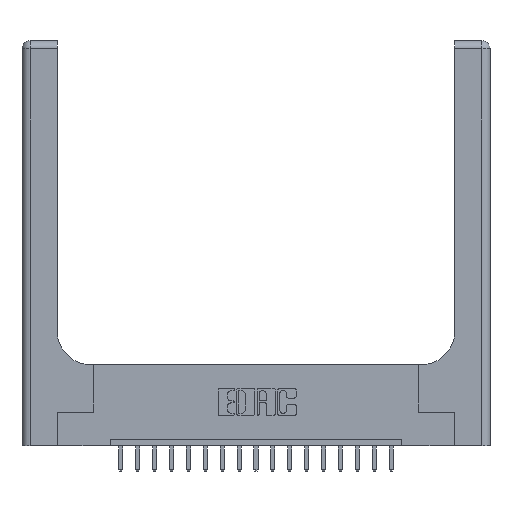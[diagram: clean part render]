
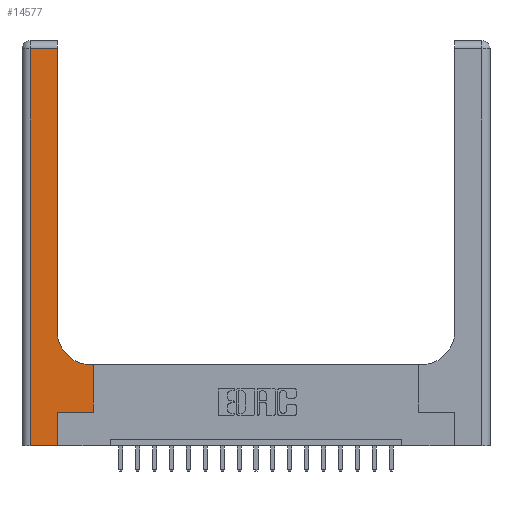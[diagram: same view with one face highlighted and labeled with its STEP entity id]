
A CAD part, top view. The second image highlights one B-rep face of the part: STEP entity #14577.
In plain terms, the highlighted planar face has unit normal (0, 0, 1).
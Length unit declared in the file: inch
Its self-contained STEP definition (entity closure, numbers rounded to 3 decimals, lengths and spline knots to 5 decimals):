
#534 = AXIS2_PLACEMENT_3D ( 'NONE', #12684, #18623, #2195 ) ;
#655 = EDGE_CURVE ( 'NONE', #13978, #4303, #18606, .T. ) ;
#719 = VECTOR ( 'NONE', #15437, 39.37008 ) ;
#831 = CARTESIAN_POINT ( 'NONE',  ( 0.26, 0.85, 0.37 ) ) ;
#1106 = EDGE_CURVE ( 'NONE', #8724, #7962, #4854, .T. ) ;
#1182 = CARTESIAN_POINT ( 'NONE',  ( 0.26, 3., 0.37 ) ) ;
#1614 = VERTEX_POINT ( 'NONE', #3201 ) ;
#1821 = VECTOR ( 'NONE', #2285, 39.37008 ) ;
#1910 = FACE_OUTER_BOUND ( 'NONE', #4806, .T. ) ;
#2195 = DIRECTION ( 'NONE',  ( -1., 0., 0. ) ) ;
#2285 = DIRECTION ( 'NONE',  ( 0., 1., 0. ) ) ;
#2563 = VECTOR ( 'NONE', #13845, 39.37008 ) ;
#2666 = ORIENTED_EDGE ( 'NONE', *, *, #9182, .T. ) ;
#3201 = CARTESIAN_POINT ( 'NONE',  ( 0.26, 2.94, 0.37 ) ) ;
#3688 = CARTESIAN_POINT ( 'NONE',  ( 0.528, 0.25, 0.37 ) ) ;
#3798 = CARTESIAN_POINT ( 'NONE',  ( 0.528, 0.6, 0.37 ) ) ;
#4148 = DIRECTION ( 'NONE',  ( 1., 0., 0. ) ) ;
#4180 = DIRECTION ( 'NONE',  ( 0., 1., 0. ) ) ;
#4295 = AXIS2_PLACEMENT_3D ( 'NONE', #17277, #9638, #14234 ) ;
#4303 = VERTEX_POINT ( 'NONE', #831 ) ;
#4405 = LINE ( 'NONE', #1182, #14149 ) ;
#4723 = CARTESIAN_POINT ( 'NONE',  ( 0.06, 0., 0.37 ) ) ;
#4806 = EDGE_LOOP ( 'NONE', ( #12585, #7739, #9282, #6896, #7894, #6172, #11822, #2666, #18138 ) ) ;
#4854 = LINE ( 'NONE', #11528, #13436 ) ;
#4890 = CARTESIAN_POINT ( 'NONE',  ( 0.06, 3., 0.37 ) ) ;
#4999 = DIRECTION ( 'NONE',  ( 0., 1., 0. ) ) ;
#5219 = EDGE_CURVE ( 'NONE', #8511, #12671, #18846, .T. ) ;
#5603 = EDGE_CURVE ( 'NONE', #11260, #8511, #8600, .T. ) ;
#5658 = CARTESIAN_POINT ( 'NONE',  ( 0.26, 0.6, 0.37 ) ) ;
#6172 = ORIENTED_EDGE ( 'NONE', *, *, #1106, .T. ) ;
#6261 = LINE ( 'NONE', #17069, #1821 ) ;
#6333 = LINE ( 'NONE', #5658, #7228 ) ;
#6896 = ORIENTED_EDGE ( 'NONE', *, *, #5219, .T. ) ;
#6936 = VECTOR ( 'NONE', #14431, 39.37008 ) ;
#7017 = EDGE_CURVE ( 'NONE', #1614, #11260, #9287, .T. ) ;
#7228 = VECTOR ( 'NONE', #19148, 39.37008 ) ;
#7581 = CARTESIAN_POINT ( 'NONE',  ( 0.06, 2.94, 0.37 ) ) ;
#7739 = ORIENTED_EDGE ( 'NONE', *, *, #7017, .T. ) ;
#7894 = ORIENTED_EDGE ( 'NONE', *, *, #15708, .T. ) ;
#7962 = VERTEX_POINT ( 'NONE', #8873 ) ;
#8511 = VERTEX_POINT ( 'NONE', #4723 ) ;
#8600 = LINE ( 'NONE', #4890, #719 ) ;
#8724 = VERTEX_POINT ( 'NONE', #10807 ) ;
#8873 = CARTESIAN_POINT ( 'NONE',  ( 0.528, 0.25, 0.37 ) ) ;
#9137 = VECTOR ( 'NONE', #4999, 39.37008 ) ;
#9182 = EDGE_CURVE ( 'NONE', #11074, #13978, #6333, .T. ) ;
#9282 = ORIENTED_EDGE ( 'NONE', *, *, #5603, .T. ) ;
#9287 = LINE ( 'NONE', #9966, #6936 ) ;
#9288 = CARTESIAN_POINT ( 'NONE',  ( 0.51, 0.6, 0.37 ) ) ;
#9589 = LINE ( 'NONE', #3688, #9137 ) ;
#9638 = DIRECTION ( 'NONE',  ( 0., 0., -1. ) ) ;
#9966 = CARTESIAN_POINT ( 'NONE',  ( 0., 2.94, 0.37 ) ) ;
#10807 = CARTESIAN_POINT ( 'NONE',  ( 0.265, 0.25, 0.37 ) ) ;
#11074 = VERTEX_POINT ( 'NONE', #3798 ) ;
#11165 = EDGE_CURVE ( 'NONE', #4303, #1614, #4405, .T. ) ;
#11260 = VERTEX_POINT ( 'NONE', #7581 ) ;
#11333 = CARTESIAN_POINT ( 'NONE',  ( 0.265, 0., 0.37 ) ) ;
#11528 = CARTESIAN_POINT ( 'NONE',  ( 0.265, 0.25, 0.37 ) ) ;
#11822 = ORIENTED_EDGE ( 'NONE', *, *, #18851, .T. ) ;
#12585 = ORIENTED_EDGE ( 'NONE', *, *, #11165, .T. ) ;
#12671 = VERTEX_POINT ( 'NONE', #11333 ) ;
#12684 = CARTESIAN_POINT ( 'NONE',  ( 0., 3., 0.37 ) ) ;
#13436 = VECTOR ( 'NONE', #4148, 39.37008 ) ;
#13845 = DIRECTION ( 'NONE',  ( 1., 0., 0. ) ) ;
#13978 = VERTEX_POINT ( 'NONE', #9288 ) ;
#14149 = VECTOR ( 'NONE', #4180, 39.37008 ) ;
#14234 = DIRECTION ( 'NONE',  ( 1., 0., 0. ) ) ;
#14431 = DIRECTION ( 'NONE',  ( -1., 0., 0. ) ) ;
#14577 = ADVANCED_FACE ( 'NONE', ( #1910 ), #15757, .F. ) ;
#15437 = DIRECTION ( 'NONE',  ( 0., -1., 0. ) ) ;
#15708 = EDGE_CURVE ( 'NONE', #12671, #8724, #6261, .T. ) ;
#15757 = PLANE ( 'NONE',  #534 ) ;
#17069 = CARTESIAN_POINT ( 'NONE',  ( 0.265, 0., 0.37 ) ) ;
#17277 = CARTESIAN_POINT ( 'NONE',  ( 0.51, 0.85, 0.37 ) ) ;
#17995 = CARTESIAN_POINT ( 'NONE',  ( 0., 0., 0.37 ) ) ;
#18138 = ORIENTED_EDGE ( 'NONE', *, *, #655, .T. ) ;
#18606 = CIRCLE ( 'NONE', #4295, 0.25 ) ;
#18623 = DIRECTION ( 'NONE',  ( 0., 0., -1. ) ) ;
#18846 = LINE ( 'NONE', #17995, #2563 ) ;
#18851 = EDGE_CURVE ( 'NONE', #7962, #11074, #9589, .T. ) ;
#19148 = DIRECTION ( 'NONE',  ( -1., 0., 0. ) ) ;
